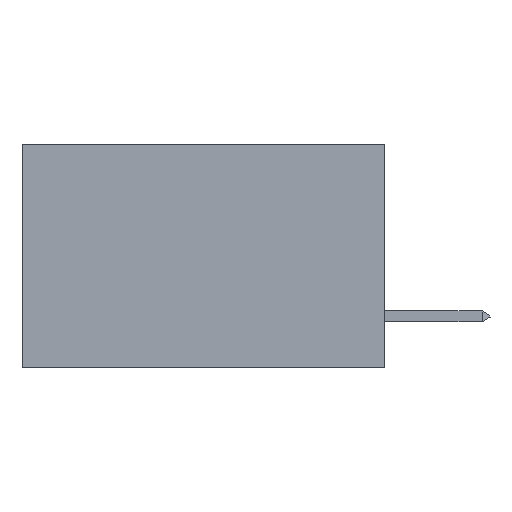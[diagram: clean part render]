
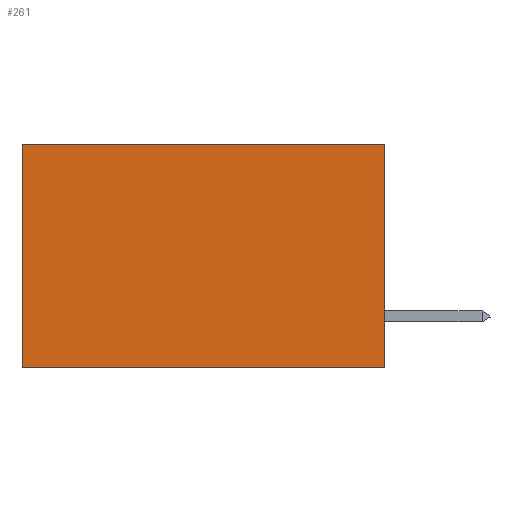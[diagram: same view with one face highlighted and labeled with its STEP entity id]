
A CAD part, left-side view. The second image highlights one B-rep face of the part: STEP entity #261.
In plain terms, the highlighted planar face has unit normal (-1, 0, 0).
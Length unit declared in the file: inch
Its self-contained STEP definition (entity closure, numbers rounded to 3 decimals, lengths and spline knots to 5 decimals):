
#261 = ADVANCED_FACE ( 'NONE', ( #18644 ), #14991, .F. ) ;
#1748 = CARTESIAN_POINT ( 'NONE',  ( 0.2875, 0.6, -0.37 ) ) ;
#2021 = VERTEX_POINT ( 'NONE', #29147 ) ;
#3543 = DIRECTION ( 'NONE',  ( 0., 1., 0. ) ) ;
#4336 = DIRECTION ( 'NONE',  ( 1., 0., 0. ) ) ;
#5168 = VECTOR ( 'NONE', #26087, 39.37008 ) ;
#6404 = LINE ( 'NONE', #24675, #32989 ) ;
#8231 = EDGE_CURVE ( 'NONE', #2021, #18547, #6404, .T. ) ;
#8428 = CARTESIAN_POINT ( 'NONE',  ( 0.2875, 0., 0. ) ) ;
#8666 = CARTESIAN_POINT ( 'NONE',  ( 0.2875, 0., 0. ) ) ;
#9860 = DIRECTION ( 'NONE',  ( 0., 0., -1. ) ) ;
#14991 = PLANE ( 'NONE',  #39429 ) ;
#15134 = DIRECTION ( 'NONE',  ( 0., 0., -1. ) ) ;
#15410 = ORIENTED_EDGE ( 'NONE', *, *, #8231, .F. ) ;
#17142 = LINE ( 'NONE', #22886, #5168 ) ;
#18547 = VERTEX_POINT ( 'NONE', #1748 ) ;
#18568 = LINE ( 'NONE', #39986, #26695 ) ;
#18577 = EDGE_CURVE ( 'NONE', #36951, #18547, #17142, .T. ) ;
#18644 = FACE_OUTER_BOUND ( 'NONE', #37083, .T. ) ;
#19177 = CARTESIAN_POINT ( 'NONE',  ( 0.2875, 0.6, 0. ) ) ;
#19699 = DIRECTION ( 'NONE',  ( 0., 1., 0. ) ) ;
#22886 = CARTESIAN_POINT ( 'NONE',  ( 0.2875, 0.6, 0. ) ) ;
#24675 = CARTESIAN_POINT ( 'NONE',  ( 0.2875, 0., -0.37 ) ) ;
#26087 = DIRECTION ( 'NONE',  ( 0., 0., -1. ) ) ;
#26695 = VECTOR ( 'NONE', #19699, 39.37008 ) ;
#28825 = EDGE_CURVE ( 'NONE', #37017, #2021, #42406, .T. ) ;
#29147 = CARTESIAN_POINT ( 'NONE',  ( 0.2875, 0., -0.37 ) ) ;
#32989 = VECTOR ( 'NONE', #3543, 39.37008 ) ;
#33448 = ORIENTED_EDGE ( 'NONE', *, *, #18577, .T. ) ;
#35708 = EDGE_CURVE ( 'NONE', #37017, #36951, #18568, .T. ) ;
#36951 = VERTEX_POINT ( 'NONE', #19177 ) ;
#37017 = VERTEX_POINT ( 'NONE', #8666 ) ;
#37083 = EDGE_LOOP ( 'NONE', ( #33448, #15410, #39438, #42927 ) ) ;
#37260 = CARTESIAN_POINT ( 'NONE',  ( 0.2875, 0., 0. ) ) ;
#39429 = AXIS2_PLACEMENT_3D ( 'NONE', #8428, #4336, #15134 ) ;
#39438 = ORIENTED_EDGE ( 'NONE', *, *, #28825, .F. ) ;
#39986 = CARTESIAN_POINT ( 'NONE',  ( 0.2875, 0., 0. ) ) ;
#41303 = VECTOR ( 'NONE', #9860, 39.37008 ) ;
#42406 = LINE ( 'NONE', #37260, #41303 ) ;
#42927 = ORIENTED_EDGE ( 'NONE', *, *, #35708, .T. ) ;
